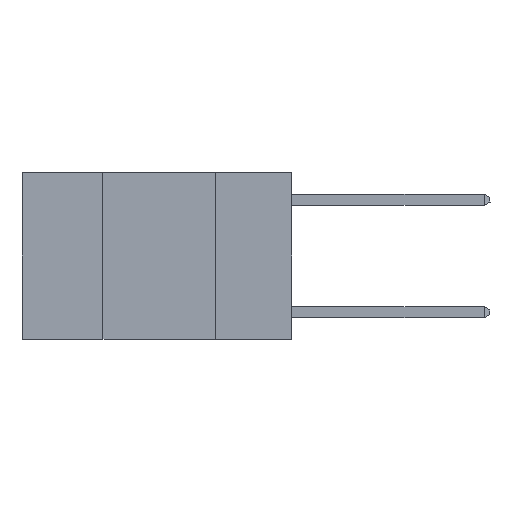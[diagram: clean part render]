
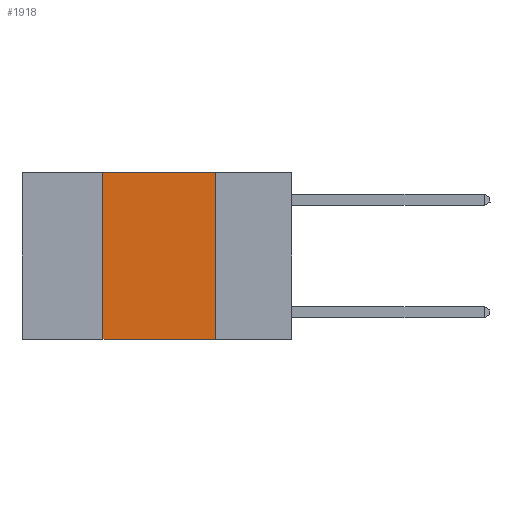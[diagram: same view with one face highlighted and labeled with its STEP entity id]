
A CAD part, left-side view. The second image highlights one B-rep face of the part: STEP entity #1918.
In plain terms, the highlighted planar face has unit normal (-1, 0, 0).
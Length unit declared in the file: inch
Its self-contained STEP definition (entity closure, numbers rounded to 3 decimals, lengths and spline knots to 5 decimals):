
#571 = EDGE_CURVE ( 'NONE', #1700, #7831, #2642, .T. ) ;
#673 = AXIS2_PLACEMENT_3D ( 'NONE', #8188, #8801, #5226 ) ;
#1082 = EDGE_CURVE ( 'NONE', #8461, #1700, #8389, .T. ) ;
#1198 = EDGE_CURVE ( 'NONE', #7831, #5232, #8099, .T. ) ;
#1231 = CARTESIAN_POINT ( 'NONE',  ( 0., 0.6, 0. ) ) ;
#1361 = EDGE_CURVE ( 'NONE', #8461, #5232, #6207, .T. ) ;
#1463 = ORIENTED_EDGE ( 'NONE', *, *, #1198, .F. ) ;
#1700 = VERTEX_POINT ( 'NONE', #4929 ) ;
#1918 = ADVANCED_FACE ( 'NONE', ( #4049 ), #3023, .F. ) ;
#2528 = EDGE_LOOP ( 'NONE', ( #1463, #7340, #7550, #4118 ) ) ;
#2642 = LINE ( 'NONE', #1231, #4449 ) ;
#2761 = CARTESIAN_POINT ( 'NONE',  ( 0., 0.17, 0. ) ) ;
#2878 = VECTOR ( 'NONE', #5817, 39.37008 ) ;
#3023 = PLANE ( 'NONE',  #673 ) ;
#3510 = VECTOR ( 'NONE', #8761, 39.37008 ) ;
#3837 = CARTESIAN_POINT ( 'NONE',  ( 0., 0.42, -0.37 ) ) ;
#4049 = FACE_OUTER_BOUND ( 'NONE', #2528, .T. ) ;
#4092 = DIRECTION ( 'NONE',  ( 0., -1., 0. ) ) ;
#4118 = ORIENTED_EDGE ( 'NONE', *, *, #1361, .T. ) ;
#4296 = VECTOR ( 'NONE', #4092, 39.37008 ) ;
#4449 = VECTOR ( 'NONE', #4792, 39.37008 ) ;
#4792 = DIRECTION ( 'NONE',  ( 0., -1., 0. ) ) ;
#4929 = CARTESIAN_POINT ( 'NONE',  ( 0., 0.42, 0. ) ) ;
#5226 = DIRECTION ( 'NONE',  ( 0., 0., -1. ) ) ;
#5232 = VERTEX_POINT ( 'NONE', #8603 ) ;
#5817 = DIRECTION ( 'NONE',  ( 0., 0., -1. ) ) ;
#6207 = LINE ( 'NONE', #8312, #4296 ) ;
#6541 = CARTESIAN_POINT ( 'NONE',  ( 0., 0.42, 0. ) ) ;
#7340 = ORIENTED_EDGE ( 'NONE', *, *, #571, .F. ) ;
#7550 = ORIENTED_EDGE ( 'NONE', *, *, #1082, .F. ) ;
#7831 = VERTEX_POINT ( 'NONE', #7985 ) ;
#7985 = CARTESIAN_POINT ( 'NONE',  ( 0., 0.17, 0. ) ) ;
#8099 = LINE ( 'NONE', #2761, #2878 ) ;
#8188 = CARTESIAN_POINT ( 'NONE',  ( 0., 0.6, 0. ) ) ;
#8312 = CARTESIAN_POINT ( 'NONE',  ( 0., 0.6, -0.37 ) ) ;
#8389 = LINE ( 'NONE', #6541, #3510 ) ;
#8461 = VERTEX_POINT ( 'NONE', #3837 ) ;
#8603 = CARTESIAN_POINT ( 'NONE',  ( 0., 0.17, -0.37 ) ) ;
#8761 = DIRECTION ( 'NONE',  ( 0., 0., 1. ) ) ;
#8801 = DIRECTION ( 'NONE',  ( 1., 0., 0. ) ) ;
